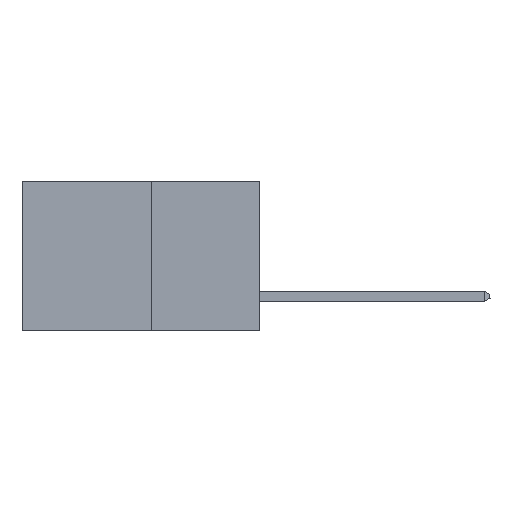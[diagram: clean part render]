
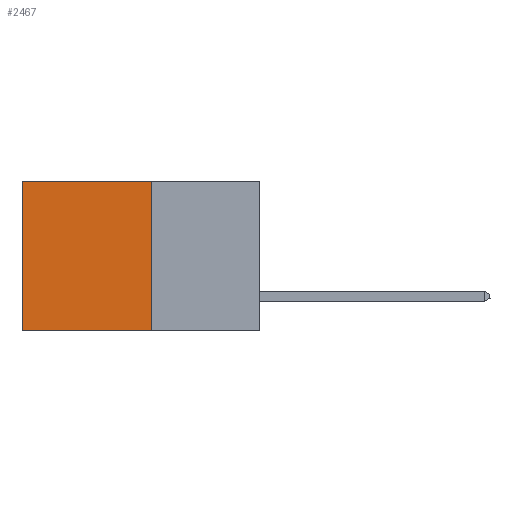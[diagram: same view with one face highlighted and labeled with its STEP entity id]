
A CAD part, left-side view. The second image highlights one B-rep face of the part: STEP entity #2467.
In plain terms, the highlighted planar face has unit normal (-1, 0, 0).
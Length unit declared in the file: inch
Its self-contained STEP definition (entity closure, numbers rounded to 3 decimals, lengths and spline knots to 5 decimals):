
#201 = ORIENTED_EDGE ( 'NONE', *, *, #3203, .F. ) ;
#908 = VERTEX_POINT ( 'NONE', #15355 ) ;
#972 = VECTOR ( 'NONE', #10792, 39.37008 ) ;
#1486 = LINE ( 'NONE', #18976, #972 ) ;
#2079 = VERTEX_POINT ( 'NONE', #4143 ) ;
#2467 = ADVANCED_FACE ( 'NONE', ( #13749 ), #9477, .F. ) ;
#3059 = LINE ( 'NONE', #17729, #20110 ) ;
#3111 = EDGE_CURVE ( 'NONE', #2079, #12709, #1486, .T. ) ;
#3203 = EDGE_CURVE ( 'NONE', #2079, #908, #8291, .T. ) ;
#3779 = CARTESIAN_POINT ( 'NONE',  ( 0.277, 0.59, -0.37 ) ) ;
#4143 = CARTESIAN_POINT ( 'NONE',  ( 0.277, 0.27, 0. ) ) ;
#4395 = VECTOR ( 'NONE', #20763, 39.37008 ) ;
#4791 = VECTOR ( 'NONE', #5474, 39.37008 ) ;
#5323 = LINE ( 'NONE', #3779, #4791 ) ;
#5474 = DIRECTION ( 'NONE',  ( 0., 0., -1. ) ) ;
#6669 = VERTEX_POINT ( 'NONE', #12362 ) ;
#7218 = ORIENTED_EDGE ( 'NONE', *, *, #3111, .T. ) ;
#8291 = LINE ( 'NONE', #15964, #4395 ) ;
#9477 = PLANE ( 'NONE',  #19461 ) ;
#10792 = DIRECTION ( 'NONE',  ( 0., 1., 0. ) ) ;
#11239 = EDGE_CURVE ( 'NONE', #12709, #6669, #5323, .T. ) ;
#12105 = EDGE_LOOP ( 'NONE', ( #18479, #17601, #201, #7218 ) ) ;
#12362 = CARTESIAN_POINT ( 'NONE',  ( 0.277, 0.59, -0.37 ) ) ;
#12709 = VERTEX_POINT ( 'NONE', #18000 ) ;
#13749 = FACE_OUTER_BOUND ( 'NONE', #12105, .T. ) ;
#14493 = DIRECTION ( 'NONE',  ( 0., 1., 0. ) ) ;
#14859 = DIRECTION ( 'NONE',  ( 1., 0., 0. ) ) ;
#15355 = CARTESIAN_POINT ( 'NONE',  ( 0.277, 0.27, -0.37 ) ) ;
#15964 = CARTESIAN_POINT ( 'NONE',  ( 0.277, 0.27, -0.37 ) ) ;
#16481 = EDGE_CURVE ( 'NONE', #908, #6669, #3059, .T. ) ;
#16757 = DIRECTION ( 'NONE',  ( 0., 0., -1. ) ) ;
#17601 = ORIENTED_EDGE ( 'NONE', *, *, #16481, .F. ) ;
#17729 = CARTESIAN_POINT ( 'NONE',  ( 0.277, 0.27, -0.37 ) ) ;
#18000 = CARTESIAN_POINT ( 'NONE',  ( 0.277, 0.59, 0. ) ) ;
#18479 = ORIENTED_EDGE ( 'NONE', *, *, #11239, .T. ) ;
#18976 = CARTESIAN_POINT ( 'NONE',  ( 0.277, 0.27, 0. ) ) ;
#19461 = AXIS2_PLACEMENT_3D ( 'NONE', #20306, #14859, #16757 ) ;
#20110 = VECTOR ( 'NONE', #14493, 39.37008 ) ;
#20306 = CARTESIAN_POINT ( 'NONE',  ( 0.277, 0.27, -0.37 ) ) ;
#20763 = DIRECTION ( 'NONE',  ( 0., 0., -1. ) ) ;
